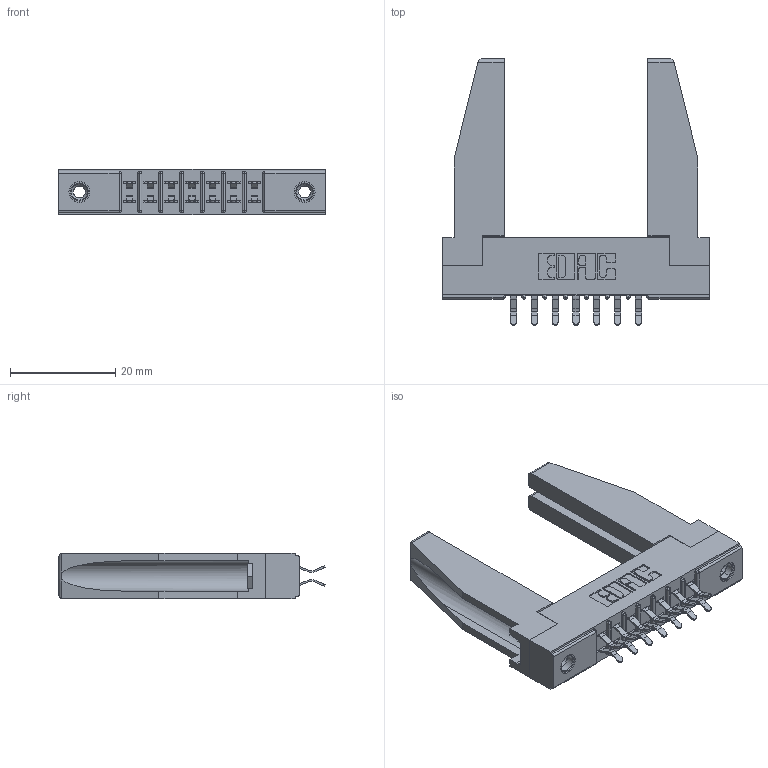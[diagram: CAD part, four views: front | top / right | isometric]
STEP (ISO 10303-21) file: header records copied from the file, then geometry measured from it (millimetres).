
FILE_DESCRIPTION (( 'STEP AP203' ), '1' );
FILE_NAME ('355-014-556-278.STEP', '2019-09-11T01:40:22', ( '' ), ( '' ), 'SwSTEP 2.0', 'SolidWorks 2016', '' );
FILE_SCHEMA (( 'CONFIG_CONTROL_DESIGN' ));
Length unit declared in the file: inch
Products named in the file (5): 355-014-556-278; 345-250-001_345-250-001-102; 305 Part_.156 Dia; 305-290-001_556; 307-220-078
Assembly tree (19 placements, depth 2):
  355-014-556-278
    305 Part_.156 Dia
    305-290-001_556  x14
    345-250-001_345-250-001-102  x2
    307-220-078  x2
Bounding box: 50.75 x 50.67 x 8.71 mm (x, y, z)
Volume: 7192.9 mm3; surface area: 9000.3 mm2
Topology: 19 solids, 19 shells, 1030 faces, 2907 edges, 1890 vertices
Faces by surface type: plane 586, cylinder 400, sphere 28, cone 12, torus 4
Entity records: 14501 total; most frequent: CARTESIAN_POINT 2409, ORIENTED_EDGE 2344, DIRECTION 2320, EDGE_CURVE 1172, LINE 902, VECTOR 902, VERTEX_POINT 756, AXIS2_PLACEMENT_3D 709
